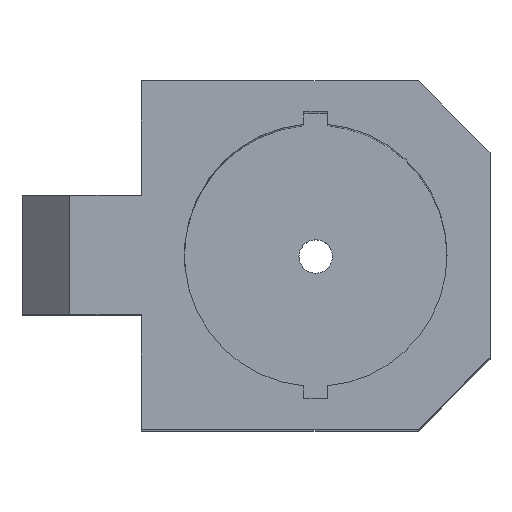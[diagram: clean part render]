
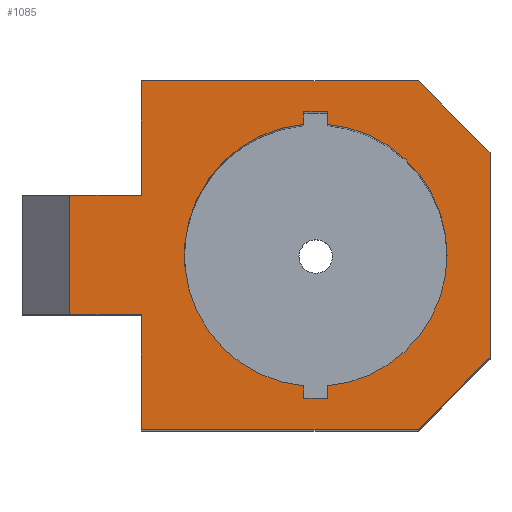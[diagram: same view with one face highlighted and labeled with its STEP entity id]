
A CAD part, top view. The second image highlights one B-rep face of the part: STEP entity #1085.
In plain terms, the highlighted planar face has unit normal (0, 0, 1).
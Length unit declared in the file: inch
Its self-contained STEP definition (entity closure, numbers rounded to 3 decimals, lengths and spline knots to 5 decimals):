
#3 = ORIENTED_EDGE ( 'NONE', *, *, #348, .T. ) ;
#49 = CARTESIAN_POINT ( 'NONE',  ( 0.73, 0.73, 0. ) ) ;
#63 = AXIS2_PLACEMENT_3D ( 'NONE', #586, #1035, #484 ) ;
#91 = VERTEX_POINT ( 'NONE', #1413 ) ;
#96 = VECTOR ( 'NONE', #1072, 39.37008 ) ;
#104 = DIRECTION ( 'NONE',  ( 0., 0., 1. ) ) ;
#108 = LINE ( 'NONE', #774, #969 ) ;
#124 = CARTESIAN_POINT ( 'NONE',  ( 0.73, 0.73, 0. ) ) ;
#129 = ORIENTED_EDGE ( 'NONE', *, *, #939, .T. ) ;
#132 = EDGE_LOOP ( 'NONE', ( #3, #923, #970, #891, #648, #677, #696, #1424, #511 ) ) ;
#138 = FACE_OUTER_BOUND ( 'NONE', #219, .T. ) ;
#153 = DIRECTION ( 'NONE',  ( 0., 1., 0. ) ) ;
#159 = LINE ( 'NONE', #270, #681 ) ;
#165 = DIRECTION ( 'NONE',  ( 1., 0., 0. ) ) ;
#169 = VECTOR ( 'NONE', #498, 39.37008 ) ;
#214 = VERTEX_POINT ( 'NONE', #415 ) ;
#219 = EDGE_LOOP ( 'NONE', ( #863, #760, #469, #489, #271, #871, #831, #129, #691, #1391 ) ) ;
#229 = VECTOR ( 'NONE', #562, 39.37008 ) ;
#237 = CARTESIAN_POINT ( 'NONE',  ( 0., 1.33, 0. ) ) ;
#240 = CIRCLE ( 'NONE', #63, 0.55 ) ;
#256 = DIRECTION ( 'NONE',  ( 0., -1., 0. ) ) ;
#262 = DIRECTION ( 'NONE',  ( -0.707, 0.707, 0. ) ) ;
#270 = CARTESIAN_POINT ( 'NONE',  ( 0., 0.48, 0. ) ) ;
#271 = ORIENTED_EDGE ( 'NONE', *, *, #373, .F. ) ;
#274 = EDGE_CURVE ( 'NONE', #1136, #558, #310, .T. ) ;
#287 = DIRECTION ( 'NONE',  ( 0., 0., 1. ) ) ;
#290 = VERTEX_POINT ( 'NONE', #668 ) ;
#310 = CIRCLE ( 'NONE', #821, 0.55 ) ;
#321 = VERTEX_POINT ( 'NONE', #1247 ) ;
#339 = DIRECTION ( 'NONE',  ( 0.707, 0.707, 0. ) ) ;
#341 = CARTESIAN_POINT ( 'NONE',  ( 1.28, 0.73, 0. ) ) ;
#345 = LINE ( 'NONE', #583, #1469 ) ;
#346 = DIRECTION ( 'NONE',  ( 1., 0., 0. ) ) ;
#348 = EDGE_CURVE ( 'NONE', #860, #1086, #1115, .T. ) ;
#359 = LINE ( 'NONE', #910, #879 ) ;
#373 = EDGE_CURVE ( 'NONE', #547, #1083, #345, .T. ) ;
#407 = EDGE_CURVE ( 'NONE', #1055, #962, #784, .T. ) ;
#409 = CARTESIAN_POINT ( 'NONE',  ( 0.78, 1.33, 0. ) ) ;
#415 = CARTESIAN_POINT ( 'NONE',  ( 0.68, 1.33, 0. ) ) ;
#434 = VECTOR ( 'NONE', #256, 39.37008 ) ;
#447 = VECTOR ( 'NONE', #844, 39.37008 ) ;
#448 = CARTESIAN_POINT ( 'NONE',  ( 0., 1.46, 0. ) ) ;
#469 = ORIENTED_EDGE ( 'NONE', *, *, #1109, .F. ) ;
#483 = EDGE_CURVE ( 'NONE', #321, #1338, #1324, .T. ) ;
#484 = DIRECTION ( 'NONE',  ( 1., 0., 0. ) ) ;
#489 = ORIENTED_EDGE ( 'NONE', *, *, #743, .F. ) ;
#493 = VERTEX_POINT ( 'NONE', #927 ) ;
#498 = DIRECTION ( 'NONE',  ( 0., -1., 0. ) ) ;
#503 = EDGE_CURVE ( 'NONE', #979, #558, #1133, .T. ) ;
#508 = LINE ( 'NONE', #237, #911 ) ;
#511 = ORIENTED_EDGE ( 'NONE', *, *, #1321, .F. ) ;
#546 = FACE_BOUND ( 'NONE', #132, .T. ) ;
#547 = VERTEX_POINT ( 'NONE', #959 ) ;
#550 = DIRECTION ( 'NONE',  ( -1., 0., 0. ) ) ;
#553 = LINE ( 'NONE', #1064, #1151 ) ;
#558 = VERTEX_POINT ( 'NONE', #597 ) ;
#562 = DIRECTION ( 'NONE',  ( 1., 0., 0. ) ) ;
#563 = EDGE_CURVE ( 'NONE', #1055, #1311, #1097, .T. ) ;
#583 = CARTESIAN_POINT ( 'NONE',  ( -0.5, 0.98, 0. ) ) ;
#586 = CARTESIAN_POINT ( 'NONE',  ( 0.73, 0.73, 0. ) ) ;
#587 = CARTESIAN_POINT ( 'NONE',  ( 1.16, 1.46, 0. ) ) ;
#597 = CARTESIAN_POINT ( 'NONE',  ( 0.78, 1.27772, 0. ) ) ;
#648 = ORIENTED_EDGE ( 'NONE', *, *, #503, .T. ) ;
#654 = EDGE_CURVE ( 'NONE', #979, #214, #508, .T. ) ;
#668 = CARTESIAN_POINT ( 'NONE',  ( 0., 1.46, 0. ) ) ;
#669 = EDGE_CURVE ( 'NONE', #899, #91, #359, .T. ) ;
#677 = ORIENTED_EDGE ( 'NONE', *, *, #274, .F. ) ;
#681 = VECTOR ( 'NONE', #1162, 39.37008 ) ;
#689 = EDGE_CURVE ( 'NONE', #1338, #1136, #240, .T. ) ;
#691 = ORIENTED_EDGE ( 'NONE', *, *, #1030, .T. ) ;
#693 = DIRECTION ( 'NONE',  ( 1., 0., 0. ) ) ;
#696 = ORIENTED_EDGE ( 'NONE', *, *, #689, .F. ) ;
#712 = VERTEX_POINT ( 'NONE', #715 ) ;
#715 = CARTESIAN_POINT ( 'NONE',  ( 0.68, 1.27772, 0. ) ) ;
#743 = EDGE_CURVE ( 'NONE', #1083, #290, #553, .T. ) ;
#760 = ORIENTED_EDGE ( 'NONE', *, *, #407, .T. ) ;
#763 = LINE ( 'NONE', #1272, #434 ) ;
#767 = VECTOR ( 'NONE', #153, 39.37008 ) ;
#774 = CARTESIAN_POINT ( 'NONE',  ( 1.46, 0.3, 0. ) ) ;
#775 = CARTESIAN_POINT ( 'NONE',  ( 0., 0., 0. ) ) ;
#784 = LINE ( 'NONE', #587, #866 ) ;
#795 = CARTESIAN_POINT ( 'NONE',  ( 0.68, 0.13, 0. ) ) ;
#821 = AXIS2_PLACEMENT_3D ( 'NONE', #124, #104, #346 ) ;
#831 = ORIENTED_EDGE ( 'NONE', *, *, #669, .F. ) ;
#832 = CIRCLE ( 'NONE', #904, 0.55 ) ;
#834 = VECTOR ( 'NONE', #1476, 39.37008 ) ;
#837 = EDGE_CURVE ( 'NONE', #493, #1311, #108, .T. ) ;
#844 = DIRECTION ( 'NONE',  ( 0., -1., 0. ) ) ;
#860 = VERTEX_POINT ( 'NONE', #795 ) ;
#863 = ORIENTED_EDGE ( 'NONE', *, *, #563, .F. ) ;
#866 = VECTOR ( 'NONE', #262, 39.37008 ) ;
#871 = ORIENTED_EDGE ( 'NONE', *, *, #876, .T. ) ;
#876 = EDGE_CURVE ( 'NONE', #547, #91, #763, .T. ) ;
#879 = VECTOR ( 'NONE', #1266, 39.37008 ) ;
#891 = ORIENTED_EDGE ( 'NONE', *, *, #654, .F. ) ;
#899 = VERTEX_POINT ( 'NONE', #941 ) ;
#904 = AXIS2_PLACEMENT_3D ( 'NONE', #49, #287, #165 ) ;
#910 = CARTESIAN_POINT ( 'NONE',  ( 0., 0.48, 0. ) ) ;
#911 = VECTOR ( 'NONE', #1023, 39.37008 ) ;
#919 = EDGE_CURVE ( 'NONE', #214, #712, #1175, .T. ) ;
#921 = CARTESIAN_POINT ( 'NONE',  ( 0.68, 0., 0. ) ) ;
#923 = ORIENTED_EDGE ( 'NONE', *, *, #1294, .F. ) ;
#927 = CARTESIAN_POINT ( 'NONE',  ( 1.16, 0., 0. ) ) ;
#939 = EDGE_CURVE ( 'NONE', #899, #1330, #159, .T. ) ;
#941 = CARTESIAN_POINT ( 'NONE',  ( 0., 0.48, 0. ) ) ;
#957 = CARTESIAN_POINT ( 'NONE',  ( 0., 0., 0. ) ) ;
#959 = CARTESIAN_POINT ( 'NONE',  ( -0.3, 0.98, 0. ) ) ;
#962 = VERTEX_POINT ( 'NONE', #1184 ) ;
#964 = CARTESIAN_POINT ( 'NONE',  ( 0., 0.13, 0. ) ) ;
#969 = VECTOR ( 'NONE', #339, 39.37008 ) ;
#970 = ORIENTED_EDGE ( 'NONE', *, *, #919, .F. ) ;
#974 = VECTOR ( 'NONE', #1148, 39.37008 ) ;
#975 = CARTESIAN_POINT ( 'NONE',  ( 1.46, 1.46, 0. ) ) ;
#979 = VERTEX_POINT ( 'NONE', #409 ) ;
#993 = DIRECTION ( 'NONE',  ( 0., 0., -1. ) ) ;
#1023 = DIRECTION ( 'NONE',  ( -1., 0., 0. ) ) ;
#1030 = EDGE_CURVE ( 'NONE', #1330, #493, #1139, .T. ) ;
#1035 = DIRECTION ( 'NONE',  ( 0., 0., 1. ) ) ;
#1055 = VERTEX_POINT ( 'NONE', #1361 ) ;
#1064 = CARTESIAN_POINT ( 'NONE',  ( 0., 0.98, 0. ) ) ;
#1072 = DIRECTION ( 'NONE',  ( 1., 0., 0. ) ) ;
#1082 = DIRECTION ( 'NONE',  ( 0., -1., 0. ) ) ;
#1083 = VERTEX_POINT ( 'NONE', #1110 ) ;
#1085 = ADVANCED_FACE ( 'NONE', ( #138, #546 ), #1448, .F. ) ;
#1086 = VERTEX_POINT ( 'NONE', #1119 ) ;
#1097 = LINE ( 'NONE', #975, #1345 ) ;
#1109 = EDGE_CURVE ( 'NONE', #290, #962, #1171, .T. ) ;
#1110 = CARTESIAN_POINT ( 'NONE',  ( 0., 0.98, 0. ) ) ;
#1111 = AXIS2_PLACEMENT_3D ( 'NONE', #448, #993, #550 ) ;
#1115 = LINE ( 'NONE', #1405, #767 ) ;
#1119 = CARTESIAN_POINT ( 'NONE',  ( 0.68, 0.18228, 0. ) ) ;
#1133 = LINE ( 'NONE', #1206, #169 ) ;
#1136 = VERTEX_POINT ( 'NONE', #341 ) ;
#1139 = LINE ( 'NONE', #775, #834 ) ;
#1148 = DIRECTION ( 'NONE',  ( 0., 1., 0. ) ) ;
#1151 = VECTOR ( 'NONE', #1318, 39.37008 ) ;
#1162 = DIRECTION ( 'NONE',  ( 0., -1., 0. ) ) ;
#1171 = LINE ( 'NONE', #1243, #229 ) ;
#1175 = LINE ( 'NONE', #921, #447 ) ;
#1184 = CARTESIAN_POINT ( 'NONE',  ( 1.16, 1.46, 0. ) ) ;
#1206 = CARTESIAN_POINT ( 'NONE',  ( 0.78, 0., 0. ) ) ;
#1243 = CARTESIAN_POINT ( 'NONE',  ( 0., 1.46, 0. ) ) ;
#1247 = CARTESIAN_POINT ( 'NONE',  ( 0.78, 0.13, 0. ) ) ;
#1266 = DIRECTION ( 'NONE',  ( -1., 0., 0. ) ) ;
#1272 = CARTESIAN_POINT ( 'NONE',  ( -0.3, 1.46, 0. ) ) ;
#1294 = EDGE_CURVE ( 'NONE', #712, #1086, #832, .T. ) ;
#1308 = CARTESIAN_POINT ( 'NONE',  ( 1.46, 0.3, 0. ) ) ;
#1311 = VERTEX_POINT ( 'NONE', #1308 ) ;
#1318 = DIRECTION ( 'NONE',  ( 0., 1., 0. ) ) ;
#1321 = EDGE_CURVE ( 'NONE', #860, #321, #1329, .T. ) ;
#1324 = LINE ( 'NONE', #1415, #974 ) ;
#1329 = LINE ( 'NONE', #964, #96 ) ;
#1330 = VERTEX_POINT ( 'NONE', #957 ) ;
#1338 = VERTEX_POINT ( 'NONE', #1468 ) ;
#1345 = VECTOR ( 'NONE', #1082, 39.37008 ) ;
#1361 = CARTESIAN_POINT ( 'NONE',  ( 1.46, 1.16, 0. ) ) ;
#1391 = ORIENTED_EDGE ( 'NONE', *, *, #837, .T. ) ;
#1405 = CARTESIAN_POINT ( 'NONE',  ( 0.68, 0., 0. ) ) ;
#1413 = CARTESIAN_POINT ( 'NONE',  ( -0.3, 0.48, 0. ) ) ;
#1415 = CARTESIAN_POINT ( 'NONE',  ( 0.78, 0., 0. ) ) ;
#1424 = ORIENTED_EDGE ( 'NONE', *, *, #483, .F. ) ;
#1448 = PLANE ( 'NONE',  #1111 ) ;
#1468 = CARTESIAN_POINT ( 'NONE',  ( 0.78, 0.18228, 0. ) ) ;
#1469 = VECTOR ( 'NONE', #693, 39.37008 ) ;
#1476 = DIRECTION ( 'NONE',  ( 1., 0., 0. ) ) ;
